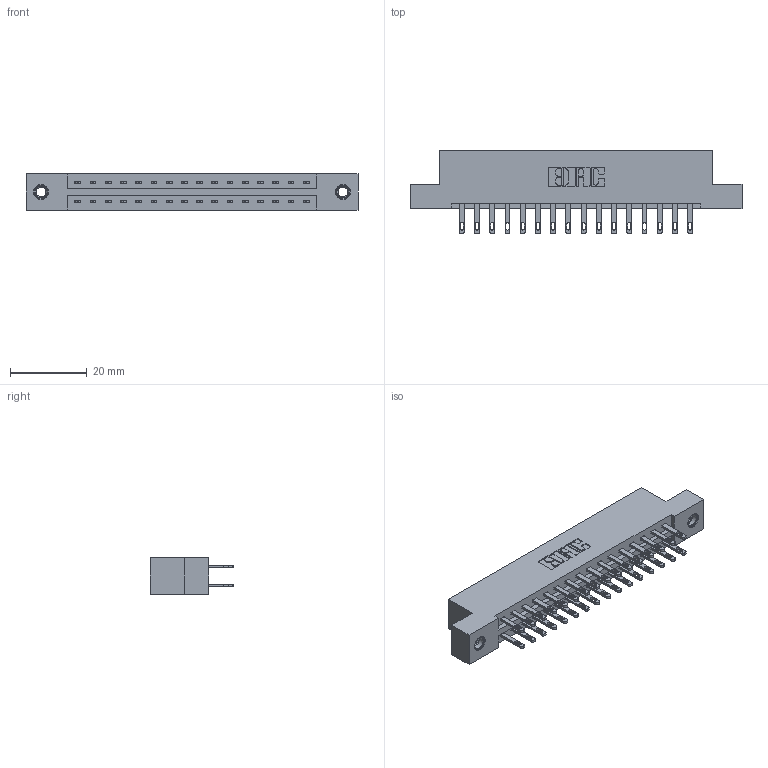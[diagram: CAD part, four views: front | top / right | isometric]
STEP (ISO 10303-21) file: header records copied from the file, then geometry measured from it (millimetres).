
FILE_DESCRIPTION (( 'STEP AP203' ), '1' );
FILE_NAME ('887-032-500-207.STEP', '2020-09-20T21:08:37', ( '' ), ( '' ), 'SwSTEP 2.0', 'SolidWorks 2020', '' );
FILE_SCHEMA (( 'CONFIG_CONTROL_DESIGN' ));
Length unit declared in the file: inch
Products named in the file (4): 887-032-500-207; 837 Part_Flush Mounting Lugs - 0.156 Dia-TI; 345-250-001_345-250-005-103; 345-292-001_345-293-100
Assembly tree (35 placements, depth 2):
  887-032-500-207
    837 Part_Flush Mounting Lugs - 0.156 Dia-TI
    345-292-001_345-293-100  x32
    345-250-001_345-250-005-103  x2
Bounding box: 86.41 x 21.85 x 9.4 mm (x, y, z)
Volume: 8844.8 mm3; surface area: 10137.6 mm2
Topology: 35 solids, 35 shells, 1774 faces, 5343 edges, 3554 vertices
Faces by surface type: plane 1126, cylinder 632, cone 12, torus 4
Entity records: 16884 total; most frequent: CARTESIAN_POINT 2845, ORIENTED_EDGE 2774, DIRECTION 2501, EDGE_CURVE 1387, VECTOR 1235, LINE 1235, VERTEX_POINT 920, AXIS2_PLACEMENT_3D 633
